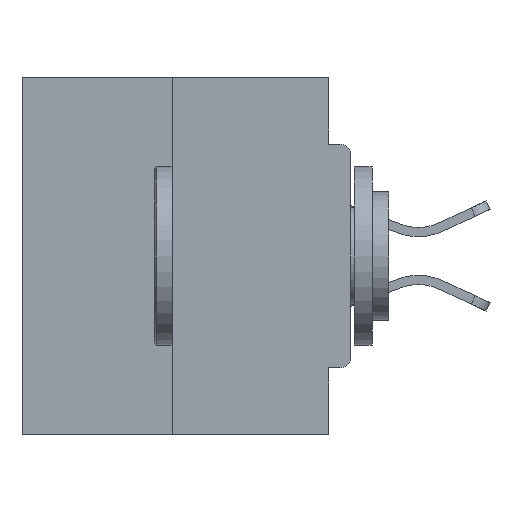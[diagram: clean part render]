
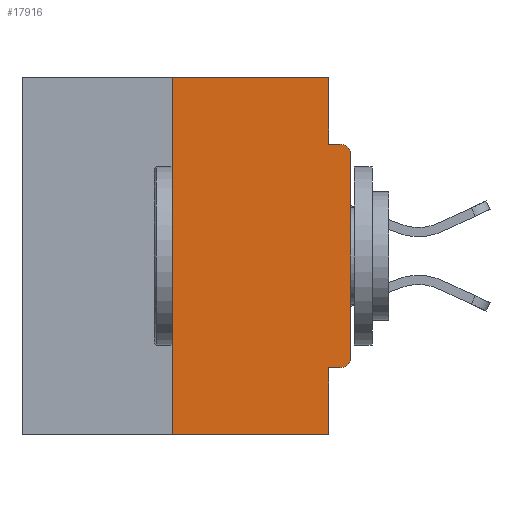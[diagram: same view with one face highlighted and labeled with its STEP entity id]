
A CAD part, left-side view. The second image highlights one B-rep face of the part: STEP entity #17916.
In plain terms, the highlighted planar face has unit normal (-1, 0, 0).
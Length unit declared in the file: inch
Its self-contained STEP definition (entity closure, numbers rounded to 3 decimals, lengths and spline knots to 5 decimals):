
#249 = CARTESIAN_POINT ( 'NONE',  ( 0., 0.031, -0.5 ) ) ;
#752 = VERTEX_POINT ( 'NONE', #27414 ) ;
#896 = EDGE_CURVE ( 'NONE', #25013, #34851, #24809, .T. ) ;
#1729 = CARTESIAN_POINT ( 'NONE',  ( 0., 0.25, 0. ) ) ;
#2412 = EDGE_CURVE ( 'NONE', #12290, #35649, #4749, .T. ) ;
#3084 = CARTESIAN_POINT ( 'NONE',  ( 0., 0.46, -0.5 ) ) ;
#3267 = DIRECTION ( 'NONE',  ( 1., 0., 0. ) ) ;
#3622 = DIRECTION ( 'NONE',  ( 0., -1., 0. ) ) ;
#3828 = DIRECTION ( 'NONE',  ( 0., 0., -1. ) ) ;
#3961 = LINE ( 'NONE', #4970, #12283 ) ;
#4749 = LINE ( 'NONE', #3084, #6428 ) ;
#4970 = CARTESIAN_POINT ( 'NONE',  ( 0., 0.46, 0. ) ) ;
#5847 = VECTOR ( 'NONE', #35126, 39.37008 ) ;
#6428 = VECTOR ( 'NONE', #10349, 39.37008 ) ;
#7391 = AXIS2_PLACEMENT_3D ( 'NONE', #41588, #45257, #34482 ) ;
#7517 = EDGE_CURVE ( 'NONE', #752, #34851, #13695, .T. ) ;
#7796 = CARTESIAN_POINT ( 'NONE',  ( 0., 0., -0.3915 ) ) ;
#8398 = LINE ( 'NONE', #35947, #41574 ) ;
#9402 = CARTESIAN_POINT ( 'NONE',  ( 0., 0.015, -0.0935 ) ) ;
#9463 = VERTEX_POINT ( 'NONE', #1729 ) ;
#10349 = DIRECTION ( 'NONE',  ( 0., -1., 0. ) ) ;
#10435 = CARTESIAN_POINT ( 'NONE',  ( 0., 0., -0.0935 ) ) ;
#10846 = CARTESIAN_POINT ( 'NONE',  ( 0., 0.031, -0.4065 ) ) ;
#11360 = DIRECTION ( 'NONE',  ( 0., 1., 0. ) ) ;
#11779 = CARTESIAN_POINT ( 'NONE',  ( 0., 0.031, 0. ) ) ;
#12283 = VECTOR ( 'NONE', #40536, 39.37008 ) ;
#12290 = VERTEX_POINT ( 'NONE', #15553 ) ;
#12359 = EDGE_LOOP ( 'NONE', ( #19218, #29269, #35158, #37428, #31272, #33519, #31039, #19437, #15347, #25978 ) ) ;
#13695 = CIRCLE ( 'NONE', #7391, 0.015 ) ;
#13951 = CARTESIAN_POINT ( 'NONE',  ( 0., 0.46, 0. ) ) ;
#14239 = EDGE_CURVE ( 'NONE', #9463, #41829, #3961, .T. ) ;
#15347 = ORIENTED_EDGE ( 'NONE', *, *, #896, .F. ) ;
#15553 = CARTESIAN_POINT ( 'NONE',  ( 0., 0.25, -0.5 ) ) ;
#16139 = FACE_OUTER_BOUND ( 'NONE', #12359, .T. ) ;
#16985 = CARTESIAN_POINT ( 'NONE',  ( 0., 0.015, -0.4065 ) ) ;
#17299 = CARTESIAN_POINT ( 'NONE',  ( 0., 0.031, 0. ) ) ;
#17472 = EDGE_CURVE ( 'NONE', #17968, #35649, #38260, .T. ) ;
#17916 = ADVANCED_FACE ( 'NONE', ( #16139 ), #44958, .F. ) ;
#17968 = VERTEX_POINT ( 'NONE', #10846 ) ;
#18975 = VERTEX_POINT ( 'NONE', #16985 ) ;
#19199 = LINE ( 'NONE', #21831, #34142 ) ;
#19218 = ORIENTED_EDGE ( 'NONE', *, *, #14239, .F. ) ;
#19437 = ORIENTED_EDGE ( 'NONE', *, *, #7517, .T. ) ;
#20832 = EDGE_CURVE ( 'NONE', #12290, #9463, #19199, .T. ) ;
#21831 = CARTESIAN_POINT ( 'NONE',  ( 0., 0.25, 0. ) ) ;
#22246 = DIRECTION ( 'NONE',  ( 0., 0., 1. ) ) ;
#23328 = EDGE_CURVE ( 'NONE', #18975, #32369, #30298, .T. ) ;
#24110 = CARTESIAN_POINT ( 'NONE',  ( 0., 0., 0. ) ) ;
#24125 = DIRECTION ( 'NONE',  ( 0., 0., -1. ) ) ;
#24384 = DIRECTION ( 'NONE',  ( 0., 0., -1. ) ) ;
#24809 = LINE ( 'NONE', #10435, #27541 ) ;
#25013 = VERTEX_POINT ( 'NONE', #41930 ) ;
#25201 = LINE ( 'NONE', #24110, #5847 ) ;
#25978 = ORIENTED_EDGE ( 'NONE', *, *, #38527, .F. ) ;
#26370 = LINE ( 'NONE', #17299, #29697 ) ;
#27172 = DIRECTION ( 'NONE',  ( 0., 0., -1. ) ) ;
#27414 = CARTESIAN_POINT ( 'NONE',  ( 0., 0., -0.1085 ) ) ;
#27541 = VECTOR ( 'NONE', #3622, 39.37008 ) ;
#29269 = ORIENTED_EDGE ( 'NONE', *, *, #20832, .F. ) ;
#29697 = VECTOR ( 'NONE', #24384, 39.37008 ) ;
#30298 = CIRCLE ( 'NONE', #44525, 0.015 ) ;
#30572 = DIRECTION ( 'NONE',  ( -1., 0., 0. ) ) ;
#31038 = VECTOR ( 'NONE', #3828, 39.37008 ) ;
#31039 = ORIENTED_EDGE ( 'NONE', *, *, #40035, .T. ) ;
#31272 = ORIENTED_EDGE ( 'NONE', *, *, #35566, .F. ) ;
#32369 = VERTEX_POINT ( 'NONE', #7796 ) ;
#33519 = ORIENTED_EDGE ( 'NONE', *, *, #23328, .T. ) ;
#34142 = VECTOR ( 'NONE', #22246, 39.37008 ) ;
#34482 = DIRECTION ( 'NONE',  ( 0., 0., -1. ) ) ;
#34851 = VERTEX_POINT ( 'NONE', #9402 ) ;
#35126 = DIRECTION ( 'NONE',  ( 0., 0., 1. ) ) ;
#35158 = ORIENTED_EDGE ( 'NONE', *, *, #2412, .T. ) ;
#35566 = EDGE_CURVE ( 'NONE', #18975, #17968, #8398, .T. ) ;
#35649 = VERTEX_POINT ( 'NONE', #43026 ) ;
#35947 = CARTESIAN_POINT ( 'NONE',  ( 0., 0., -0.4065 ) ) ;
#37428 = ORIENTED_EDGE ( 'NONE', *, *, #17472, .F. ) ;
#38260 = LINE ( 'NONE', #249, #31038 ) ;
#38461 = AXIS2_PLACEMENT_3D ( 'NONE', #13951, #3267, #24125 ) ;
#38527 = EDGE_CURVE ( 'NONE', #41829, #25013, #26370, .T. ) ;
#40035 = EDGE_CURVE ( 'NONE', #32369, #752, #25201, .T. ) ;
#40536 = DIRECTION ( 'NONE',  ( 0., -1., 0. ) ) ;
#41574 = VECTOR ( 'NONE', #11360, 39.37008 ) ;
#41588 = CARTESIAN_POINT ( 'NONE',  ( 0., 0.015, -0.1085 ) ) ;
#41829 = VERTEX_POINT ( 'NONE', #11779 ) ;
#41930 = CARTESIAN_POINT ( 'NONE',  ( 0., 0.031, -0.0935 ) ) ;
#43026 = CARTESIAN_POINT ( 'NONE',  ( 0., 0.031, -0.5 ) ) ;
#44525 = AXIS2_PLACEMENT_3D ( 'NONE', #45082, #30572, #27172 ) ;
#44958 = PLANE ( 'NONE',  #38461 ) ;
#45082 = CARTESIAN_POINT ( 'NONE',  ( 0., 0.015, -0.3915 ) ) ;
#45257 = DIRECTION ( 'NONE',  ( -1., 0., 0. ) ) ;
